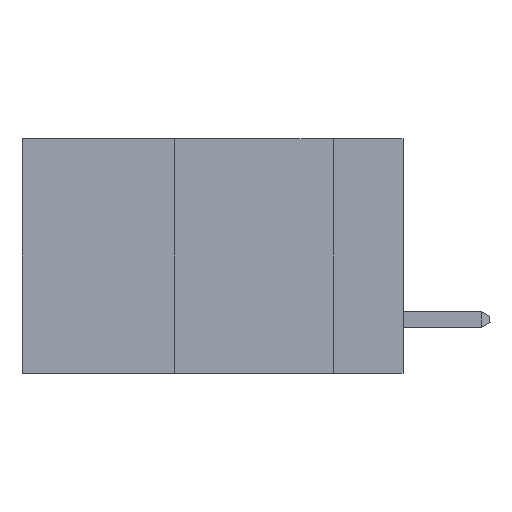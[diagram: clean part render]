
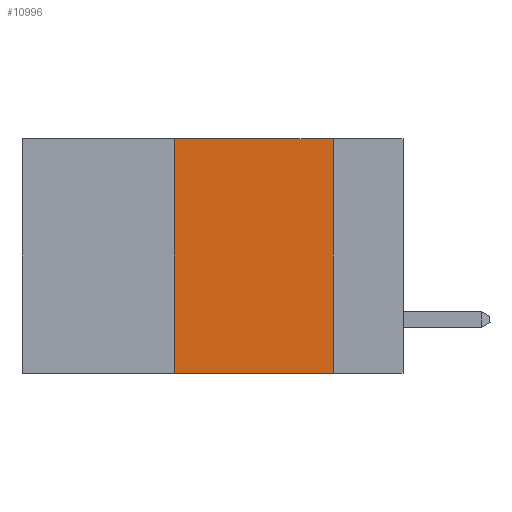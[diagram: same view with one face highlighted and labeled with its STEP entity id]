
A CAD part, left-side view. The second image highlights one B-rep face of the part: STEP entity #10996.
In plain terms, the highlighted planar face has unit normal (-1, 0, 0).
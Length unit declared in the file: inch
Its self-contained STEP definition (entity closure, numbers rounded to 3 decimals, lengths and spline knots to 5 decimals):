
#416 = ORIENTED_EDGE ( 'NONE', *, *, #23591, .F. ) ;
#550 = DIRECTION ( 'NONE',  ( 0., -1., 0. ) ) ;
#909 = DIRECTION ( 'NONE',  ( 1., 0., 0. ) ) ;
#1700 = CARTESIAN_POINT ( 'NONE',  ( 0., 0.36, 0. ) ) ;
#1837 = EDGE_LOOP ( 'NONE', ( #31104, #416, #22481, #33883 ) ) ;
#3592 = LINE ( 'NONE', #32062, #19214 ) ;
#3785 = LINE ( 'NONE', #5628, #34047 ) ;
#3810 = VERTEX_POINT ( 'NONE', #37661 ) ;
#5452 = LINE ( 'NONE', #1700, #35641 ) ;
#5628 = CARTESIAN_POINT ( 'NONE',  ( 0., 0.6, -0.37 ) ) ;
#6335 = CARTESIAN_POINT ( 'NONE',  ( 0., 0.11, -0.37 ) ) ;
#10996 = ADVANCED_FACE ( 'NONE', ( #17658 ), #15613, .F. ) ;
#11638 = CARTESIAN_POINT ( 'NONE',  ( 0., 0.6, 0. ) ) ;
#11883 = AXIS2_PLACEMENT_3D ( 'NONE', #35996, #909, #21437 ) ;
#12652 = VERTEX_POINT ( 'NONE', #19841 ) ;
#13239 = VERTEX_POINT ( 'NONE', #34137 ) ;
#14741 = EDGE_CURVE ( 'NONE', #13239, #34119, #3785, .T. ) ;
#15613 = PLANE ( 'NONE',  #11883 ) ;
#16200 = LINE ( 'NONE', #11638, #33551 ) ;
#17658 = FACE_OUTER_BOUND ( 'NONE', #1837, .T. ) ;
#19214 = VECTOR ( 'NONE', #26265, 39.37008 ) ;
#19841 = CARTESIAN_POINT ( 'NONE',  ( 0., 0.11, 0. ) ) ;
#20447 = EDGE_CURVE ( 'NONE', #13239, #3810, #5452, .T. ) ;
#21437 = DIRECTION ( 'NONE',  ( 0., 0., -1. ) ) ;
#22481 = ORIENTED_EDGE ( 'NONE', *, *, #20447, .F. ) ;
#23591 = EDGE_CURVE ( 'NONE', #3810, #12652, #16200, .T. ) ;
#25108 = DIRECTION ( 'NONE',  ( 0., 0., 1. ) ) ;
#25413 = EDGE_CURVE ( 'NONE', #12652, #34119, #3592, .T. ) ;
#26265 = DIRECTION ( 'NONE',  ( 0., 0., -1. ) ) ;
#31104 = ORIENTED_EDGE ( 'NONE', *, *, #25413, .F. ) ;
#32052 = DIRECTION ( 'NONE',  ( 0., -1., 0. ) ) ;
#32062 = CARTESIAN_POINT ( 'NONE',  ( 0., 0.11, 0. ) ) ;
#33551 = VECTOR ( 'NONE', #32052, 39.37008 ) ;
#33883 = ORIENTED_EDGE ( 'NONE', *, *, #14741, .T. ) ;
#34047 = VECTOR ( 'NONE', #550, 39.37008 ) ;
#34119 = VERTEX_POINT ( 'NONE', #6335 ) ;
#34137 = CARTESIAN_POINT ( 'NONE',  ( 0., 0.36, -0.37 ) ) ;
#35641 = VECTOR ( 'NONE', #25108, 39.37008 ) ;
#35996 = CARTESIAN_POINT ( 'NONE',  ( 0., 0.6, 0. ) ) ;
#37661 = CARTESIAN_POINT ( 'NONE',  ( 0., 0.36, 0. ) ) ;
